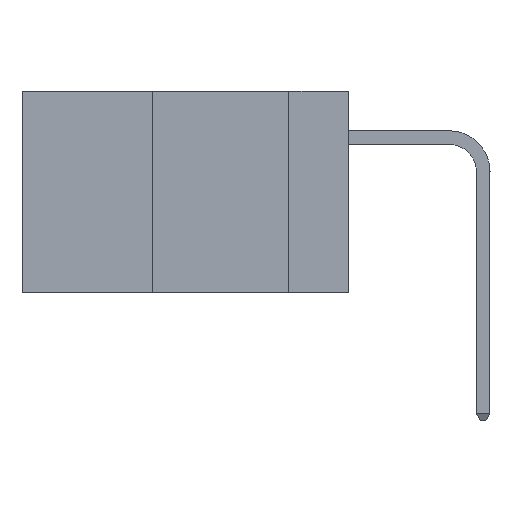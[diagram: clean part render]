
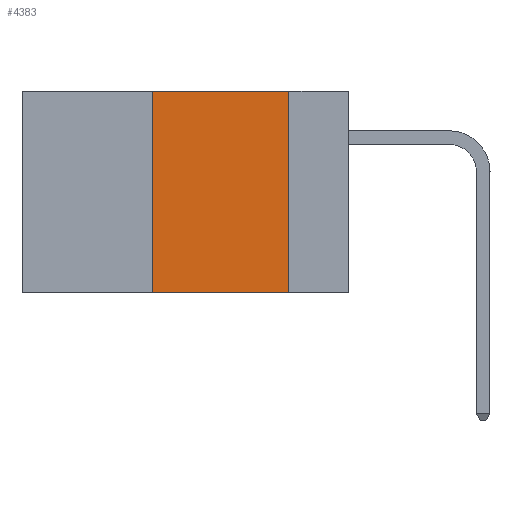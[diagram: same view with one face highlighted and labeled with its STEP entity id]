
A CAD part, left-side view. The second image highlights one B-rep face of the part: STEP entity #4383.
In plain terms, the highlighted planar face has unit normal (-1, 0, 0).
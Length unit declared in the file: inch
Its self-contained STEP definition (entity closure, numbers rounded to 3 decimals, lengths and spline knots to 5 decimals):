
#1207 = VECTOR ( 'NONE', #21992, 39.37008 ) ;
#1357 = VECTOR ( 'NONE', #7634, 39.37008 ) ;
#1629 = EDGE_CURVE ( 'NONE', #28915, #17424, #9407, .T. ) ;
#1739 = VECTOR ( 'NONE', #2859, 39.37008 ) ;
#2859 = DIRECTION ( 'NONE',  ( 0., -1., 0. ) ) ;
#3485 = CARTESIAN_POINT ( 'NONE',  ( 0., 0.36, 0. ) ) ;
#4271 = ORIENTED_EDGE ( 'NONE', *, *, #38042, .F. ) ;
#4383 = ADVANCED_FACE ( 'NONE', ( #12477 ), #22460, .F. ) ;
#5045 = ORIENTED_EDGE ( 'NONE', *, *, #13486, .F. ) ;
#7312 = VERTEX_POINT ( 'NONE', #17710 ) ;
#7634 = DIRECTION ( 'NONE',  ( 0., -1., 0. ) ) ;
#7998 = EDGE_CURVE ( 'NONE', #7312, #17424, #10870, .T. ) ;
#8915 = CARTESIAN_POINT ( 'NONE',  ( 0., 0.6, -0.37 ) ) ;
#9407 = LINE ( 'NONE', #16180, #1207 ) ;
#10870 = LINE ( 'NONE', #8915, #1739 ) ;
#11349 = VERTEX_POINT ( 'NONE', #29034 ) ;
#12477 = FACE_OUTER_BOUND ( 'NONE', #20361, .T. ) ;
#12832 = DIRECTION ( 'NONE',  ( 0., 0., 1. ) ) ;
#13486 = EDGE_CURVE ( 'NONE', #7312, #11349, #33610, .T. ) ;
#13508 = ORIENTED_EDGE ( 'NONE', *, *, #7998, .T. ) ;
#15126 = CARTESIAN_POINT ( 'NONE',  ( 0., 0.6, 0. ) ) ;
#16180 = CARTESIAN_POINT ( 'NONE',  ( 0., 0.11, 0. ) ) ;
#16599 = DIRECTION ( 'NONE',  ( 0., 0., -1. ) ) ;
#17386 = AXIS2_PLACEMENT_3D ( 'NONE', #15126, #26586, #16599 ) ;
#17424 = VERTEX_POINT ( 'NONE', #19152 ) ;
#17710 = CARTESIAN_POINT ( 'NONE',  ( 0., 0.36, -0.37 ) ) ;
#19152 = CARTESIAN_POINT ( 'NONE',  ( 0., 0.11, -0.37 ) ) ;
#20361 = EDGE_LOOP ( 'NONE', ( #26469, #4271, #5045, #13508 ) ) ;
#21992 = DIRECTION ( 'NONE',  ( 0., 0., -1. ) ) ;
#22460 = PLANE ( 'NONE',  #17386 ) ;
#22776 = CARTESIAN_POINT ( 'NONE',  ( 0., 0.11, 0. ) ) ;
#25877 = VECTOR ( 'NONE', #12832, 39.37008 ) ;
#26469 = ORIENTED_EDGE ( 'NONE', *, *, #1629, .F. ) ;
#26586 = DIRECTION ( 'NONE',  ( 1., 0., 0. ) ) ;
#28915 = VERTEX_POINT ( 'NONE', #22776 ) ;
#29034 = CARTESIAN_POINT ( 'NONE',  ( 0., 0.36, 0. ) ) ;
#31236 = CARTESIAN_POINT ( 'NONE',  ( 0., 0.6, 0. ) ) ;
#32110 = LINE ( 'NONE', #31236, #1357 ) ;
#33610 = LINE ( 'NONE', #3485, #25877 ) ;
#38042 = EDGE_CURVE ( 'NONE', #11349, #28915, #32110, .T. ) ;
